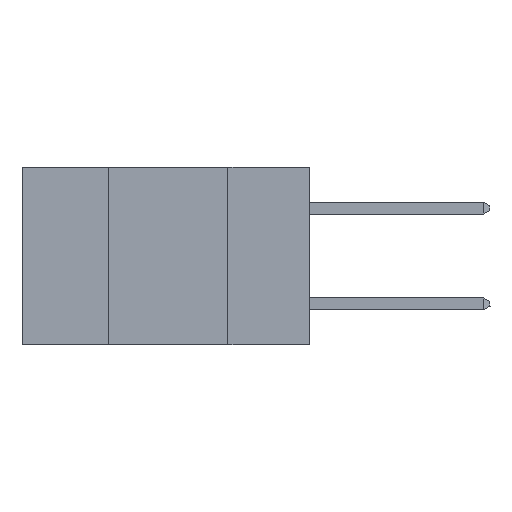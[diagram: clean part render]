
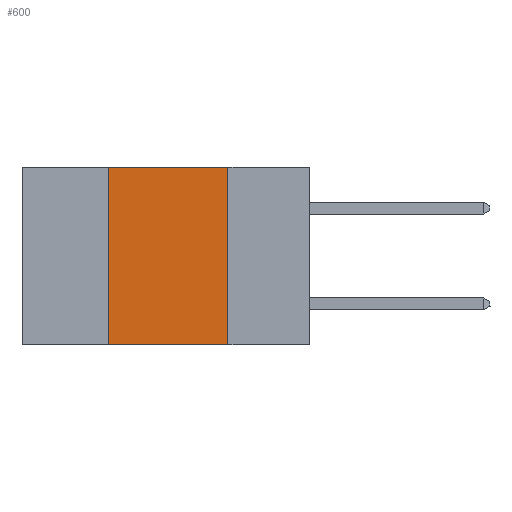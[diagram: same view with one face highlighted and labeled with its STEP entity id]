
A CAD part, left-side view. The second image highlights one B-rep face of the part: STEP entity #600.
In plain terms, the highlighted planar face has unit normal (-1, 0, 0).
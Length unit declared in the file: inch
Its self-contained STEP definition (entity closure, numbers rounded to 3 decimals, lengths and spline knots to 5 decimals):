
#600 = ADVANCED_FACE ( 'NONE', ( #11763 ), #5691, .F. ) ;
#708 = VERTEX_POINT ( 'NONE', #2778 ) ;
#903 = DIRECTION ( 'NONE',  ( 0., -1., 0. ) ) ;
#947 = CARTESIAN_POINT ( 'NONE',  ( 0., 0.6, 0. ) ) ;
#1080 = VECTOR ( 'NONE', #10262, 39.37008 ) ;
#1258 = DIRECTION ( 'NONE',  ( 0., 0., 1. ) ) ;
#1668 = VERTEX_POINT ( 'NONE', #2862 ) ;
#1775 = VERTEX_POINT ( 'NONE', #6158 ) ;
#1808 = EDGE_CURVE ( 'NONE', #1775, #708, #1939, .T. ) ;
#1900 = LINE ( 'NONE', #8604, #12618 ) ;
#1939 = LINE ( 'NONE', #4098, #4463 ) ;
#2778 = CARTESIAN_POINT ( 'NONE',  ( 0., 0.17, -0.37 ) ) ;
#2862 = CARTESIAN_POINT ( 'NONE',  ( 0., 0.17, 0. ) ) ;
#3290 = EDGE_CURVE ( 'NONE', #1775, #7154, #1900, .T. ) ;
#3915 = VECTOR ( 'NONE', #8674, 39.37008 ) ;
#3980 = EDGE_CURVE ( 'NONE', #1668, #708, #6688, .T. ) ;
#4081 = CARTESIAN_POINT ( 'NONE',  ( 0., 0.6, 0. ) ) ;
#4098 = CARTESIAN_POINT ( 'NONE',  ( 0., 0.6, -0.37 ) ) ;
#4463 = VECTOR ( 'NONE', #903, 39.37008 ) ;
#5361 = ORIENTED_EDGE ( 'NONE', *, *, #3290, .F. ) ;
#5691 = PLANE ( 'NONE',  #9044 ) ;
#6158 = CARTESIAN_POINT ( 'NONE',  ( 0., 0.42, -0.37 ) ) ;
#6610 = CARTESIAN_POINT ( 'NONE',  ( 0., 0.17, 0. ) ) ;
#6688 = LINE ( 'NONE', #6610, #3915 ) ;
#7154 = VERTEX_POINT ( 'NONE', #10607 ) ;
#7426 = ORIENTED_EDGE ( 'NONE', *, *, #1808, .T. ) ;
#8180 = DIRECTION ( 'NONE',  ( 0., 0., -1. ) ) ;
#8604 = CARTESIAN_POINT ( 'NONE',  ( 0., 0.42, 0. ) ) ;
#8674 = DIRECTION ( 'NONE',  ( 0., 0., -1. ) ) ;
#8762 = EDGE_CURVE ( 'NONE', #7154, #1668, #11553, .T. ) ;
#8799 = ORIENTED_EDGE ( 'NONE', *, *, #3980, .F. ) ;
#8801 = ORIENTED_EDGE ( 'NONE', *, *, #8762, .F. ) ;
#9044 = AXIS2_PLACEMENT_3D ( 'NONE', #947, #10580, #8180 ) ;
#10262 = DIRECTION ( 'NONE',  ( 0., -1., 0. ) ) ;
#10580 = DIRECTION ( 'NONE',  ( 1., 0., 0. ) ) ;
#10607 = CARTESIAN_POINT ( 'NONE',  ( 0., 0.42, 0. ) ) ;
#10856 = EDGE_LOOP ( 'NONE', ( #8799, #8801, #5361, #7426 ) ) ;
#11553 = LINE ( 'NONE', #4081, #1080 ) ;
#11763 = FACE_OUTER_BOUND ( 'NONE', #10856, .T. ) ;
#12618 = VECTOR ( 'NONE', #1258, 39.37008 ) ;
